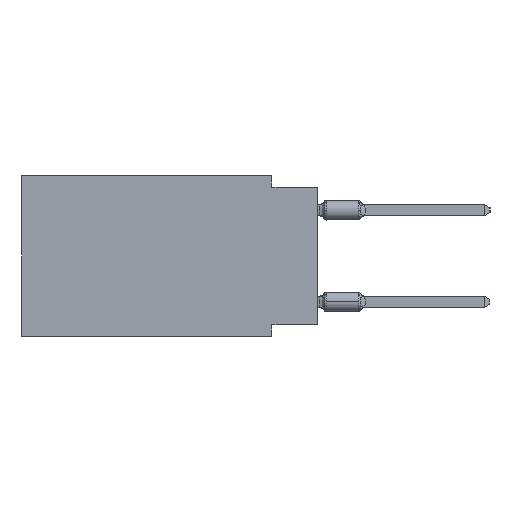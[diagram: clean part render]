
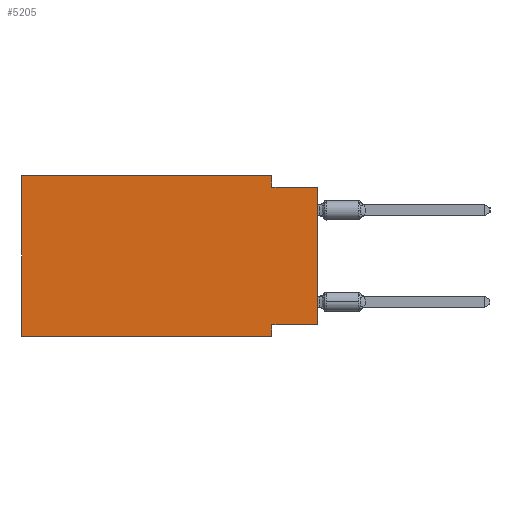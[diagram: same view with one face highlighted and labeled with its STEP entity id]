
A CAD part, left-side view. The second image highlights one B-rep face of the part: STEP entity #5205.
In plain terms, the highlighted planar face has unit normal (-1, 0, 0).
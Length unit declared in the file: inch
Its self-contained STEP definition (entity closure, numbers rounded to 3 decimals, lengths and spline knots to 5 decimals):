
#144 = CARTESIAN_POINT ( 'NONE',  ( 0., 0.645, -0.35 ) ) ;
#937 = DIRECTION ( 'NONE',  ( 0., -1., 0. ) ) ;
#1762 = CARTESIAN_POINT ( 'NONE',  ( 0., 0.1, 0. ) ) ;
#2860 = EDGE_CURVE ( 'NONE', #37645, #44762, #36486, .T. ) ;
#3595 = DIRECTION ( 'NONE',  ( 0., -1., 0. ) ) ;
#4335 = DIRECTION ( 'NONE',  ( 1., 0., 0. ) ) ;
#5205 = ADVANCED_FACE ( 'NONE', ( #15825 ), #5295, .F. ) ;
#5295 = PLANE ( 'NONE',  #9184 ) ;
#5452 = CARTESIAN_POINT ( 'NONE',  ( 0., 0.645, 0. ) ) ;
#7075 = VECTOR ( 'NONE', #44924, 39.37008 ) ;
#8460 = VERTEX_POINT ( 'NONE', #5452 ) ;
#8856 = VECTOR ( 'NONE', #3595, 39.37008 ) ;
#9184 = AXIS2_PLACEMENT_3D ( 'NONE', #16550, #4335, #19983 ) ;
#9542 = EDGE_CURVE ( 'NONE', #37645, #14374, #38741, .T. ) ;
#9841 = DIRECTION ( 'NONE',  ( 0., 0., 1. ) ) ;
#10024 = ORIENTED_EDGE ( 'NONE', *, *, #24001, .T. ) ;
#10412 = VERTEX_POINT ( 'NONE', #19076 ) ;
#10434 = LINE ( 'NONE', #35899, #22673 ) ;
#13115 = CARTESIAN_POINT ( 'NONE',  ( 0., 0.1, -0.325 ) ) ;
#14374 = VERTEX_POINT ( 'NONE', #13115 ) ;
#14989 = ORIENTED_EDGE ( 'NONE', *, *, #46904, .F. ) ;
#15169 = VERTEX_POINT ( 'NONE', #44835 ) ;
#15602 = CARTESIAN_POINT ( 'NONE',  ( 0., 0.1, 0. ) ) ;
#15825 = FACE_OUTER_BOUND ( 'NONE', #46027, .T. ) ;
#16550 = CARTESIAN_POINT ( 'NONE',  ( 0., 0.645, 0. ) ) ;
#16614 = EDGE_CURVE ( 'NONE', #15169, #44762, #37105, .T. ) ;
#16928 = ORIENTED_EDGE ( 'NONE', *, *, #16614, .F. ) ;
#17472 = CARTESIAN_POINT ( 'NONE',  ( 0., 0., -0.325 ) ) ;
#17890 = CARTESIAN_POINT ( 'NONE',  ( 0., 0., 0. ) ) ;
#18271 = CARTESIAN_POINT ( 'NONE',  ( 0., 0., -0.025 ) ) ;
#19076 = CARTESIAN_POINT ( 'NONE',  ( 0., 0.645, -0.35 ) ) ;
#19983 = DIRECTION ( 'NONE',  ( 0., 0., -1. ) ) ;
#20354 = DIRECTION ( 'NONE',  ( 0., 0., -1. ) ) ;
#20448 = EDGE_CURVE ( 'NONE', #10412, #8460, #43387, .T. ) ;
#20981 = ORIENTED_EDGE ( 'NONE', *, *, #20448, .F. ) ;
#22673 = VECTOR ( 'NONE', #40057, 39.37008 ) ;
#22724 = VECTOR ( 'NONE', #20354, 39.37008 ) ;
#23576 = CARTESIAN_POINT ( 'NONE',  ( 0., 0., -0.325 ) ) ;
#24001 = EDGE_CURVE ( 'NONE', #10412, #43807, #33666, .T. ) ;
#24836 = VECTOR ( 'NONE', #937, 39.37008 ) ;
#27487 = LINE ( 'NONE', #1762, #22724 ) ;
#27649 = ORIENTED_EDGE ( 'NONE', *, *, #36165, .F. ) ;
#29927 = VECTOR ( 'NONE', #47514, 39.37008 ) ;
#30319 = LINE ( 'NONE', #34462, #24836 ) ;
#30899 = EDGE_CURVE ( 'NONE', #8460, #44096, #30319, .T. ) ;
#32455 = VECTOR ( 'NONE', #9841, 39.37008 ) ;
#33666 = LINE ( 'NONE', #144, #7075 ) ;
#34462 = CARTESIAN_POINT ( 'NONE',  ( 0., 0.645, 0. ) ) ;
#35036 = VECTOR ( 'NONE', #35313, 39.37008 ) ;
#35313 = DIRECTION ( 'NONE',  ( 0., 1., 0. ) ) ;
#35899 = CARTESIAN_POINT ( 'NONE',  ( 0., 0.1, -0.35 ) ) ;
#36165 = EDGE_CURVE ( 'NONE', #44096, #15169, #27487, .T. ) ;
#36486 = LINE ( 'NONE', #17890, #29927 ) ;
#36619 = ORIENTED_EDGE ( 'NONE', *, *, #9542, .F. ) ;
#37105 = LINE ( 'NONE', #18271, #8856 ) ;
#37645 = VERTEX_POINT ( 'NONE', #17472 ) ;
#38741 = LINE ( 'NONE', #23576, #35036 ) ;
#39454 = CARTESIAN_POINT ( 'NONE',  ( 0., 0.645, 0. ) ) ;
#40057 = DIRECTION ( 'NONE',  ( 0., 0., -1. ) ) ;
#40985 = ORIENTED_EDGE ( 'NONE', *, *, #30899, .F. ) ;
#42456 = CARTESIAN_POINT ( 'NONE',  ( 0., 0., -0.025 ) ) ;
#43387 = LINE ( 'NONE', #39454, #32455 ) ;
#43807 = VERTEX_POINT ( 'NONE', #46013 ) ;
#44096 = VERTEX_POINT ( 'NONE', #15602 ) ;
#44762 = VERTEX_POINT ( 'NONE', #42456 ) ;
#44835 = CARTESIAN_POINT ( 'NONE',  ( 0., 0.1, -0.025 ) ) ;
#44924 = DIRECTION ( 'NONE',  ( 0., -1., 0. ) ) ;
#45073 = ORIENTED_EDGE ( 'NONE', *, *, #2860, .T. ) ;
#46013 = CARTESIAN_POINT ( 'NONE',  ( 0., 0.1, -0.35 ) ) ;
#46027 = EDGE_LOOP ( 'NONE', ( #45073, #16928, #27649, #40985, #20981, #10024, #14989, #36619 ) ) ;
#46904 = EDGE_CURVE ( 'NONE', #14374, #43807, #10434, .T. ) ;
#47514 = DIRECTION ( 'NONE',  ( 0., 0., 1. ) ) ;
